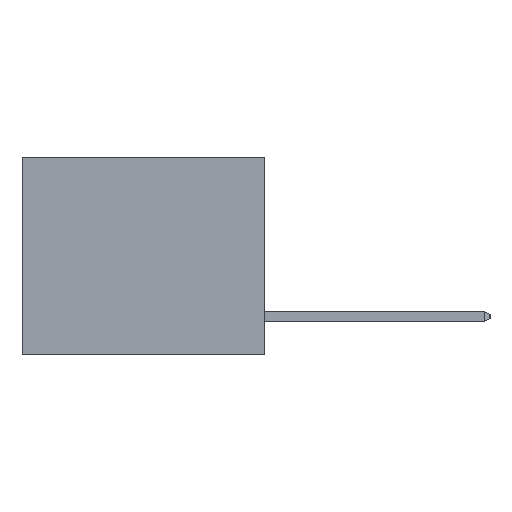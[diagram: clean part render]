
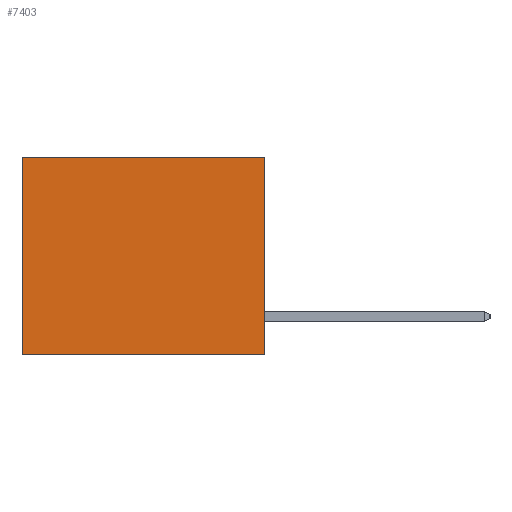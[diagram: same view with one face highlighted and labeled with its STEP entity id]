
A CAD part, left-side view. The second image highlights one B-rep face of the part: STEP entity #7403.
In plain terms, the highlighted planar face has unit normal (-1, 0, 0).
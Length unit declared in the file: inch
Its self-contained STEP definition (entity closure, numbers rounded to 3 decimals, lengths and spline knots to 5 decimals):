
#246 = AXIS2_PLACEMENT_3D ( 'NONE', #17923, #2423, #8556 ) ;
#753 = VECTOR ( 'NONE', #1639, 39.37008 ) ;
#1365 = CARTESIAN_POINT ( 'NONE',  ( 0.3165, 0., -0.49 ) ) ;
#1639 = DIRECTION ( 'NONE',  ( 0., 1., 0. ) ) ;
#1833 = CARTESIAN_POINT ( 'NONE',  ( 0.3165, 0., 0. ) ) ;
#2423 = DIRECTION ( 'NONE',  ( 1., 0., 0. ) ) ;
#2845 = CARTESIAN_POINT ( 'NONE',  ( 0.3165, 0., 0. ) ) ;
#3316 = CARTESIAN_POINT ( 'NONE',  ( 0.3165, 0.6, -0.49 ) ) ;
#3956 = VECTOR ( 'NONE', #10440, 39.37008 ) ;
#4704 = CARTESIAN_POINT ( 'NONE',  ( 0.3165, 0., -0.49 ) ) ;
#4845 = VERTEX_POINT ( 'NONE', #12068 ) ;
#5473 = PLANE ( 'NONE',  #246 ) ;
#5588 = ORIENTED_EDGE ( 'NONE', *, *, #15185, .T. ) ;
#6753 = EDGE_CURVE ( 'NONE', #7168, #4845, #12790, .T. ) ;
#7168 = VERTEX_POINT ( 'NONE', #2845 ) ;
#7403 = ADVANCED_FACE ( 'NONE', ( #8034 ), #5473, .F. ) ;
#7908 = LINE ( 'NONE', #1365, #19827 ) ;
#8034 = FACE_OUTER_BOUND ( 'NONE', #8090, .T. ) ;
#8090 = EDGE_LOOP ( 'NONE', ( #8591, #9976, #17441, #5588 ) ) ;
#8556 = DIRECTION ( 'NONE',  ( 0., 0., -1. ) ) ;
#8591 = ORIENTED_EDGE ( 'NONE', *, *, #18646, .T. ) ;
#8878 = CARTESIAN_POINT ( 'NONE',  ( 0.3165, 0.6, -0.49 ) ) ;
#9976 = ORIENTED_EDGE ( 'NONE', *, *, #17591, .F. ) ;
#10440 = DIRECTION ( 'NONE',  ( 0., 0., -1. ) ) ;
#12068 = CARTESIAN_POINT ( 'NONE',  ( 0.3165, 0., -0.49 ) ) ;
#12761 = VERTEX_POINT ( 'NONE', #3316 ) ;
#12790 = LINE ( 'NONE', #4704, #16690 ) ;
#15185 = EDGE_CURVE ( 'NONE', #7168, #17456, #17766, .T. ) ;
#15728 = DIRECTION ( 'NONE',  ( 0., 0., -1. ) ) ;
#15958 = CARTESIAN_POINT ( 'NONE',  ( 0.3165, 0.6, 0. ) ) ;
#16690 = VECTOR ( 'NONE', #15728, 39.37008 ) ;
#17441 = ORIENTED_EDGE ( 'NONE', *, *, #6753, .F. ) ;
#17456 = VERTEX_POINT ( 'NONE', #15958 ) ;
#17591 = EDGE_CURVE ( 'NONE', #4845, #12761, #7908, .T. ) ;
#17766 = LINE ( 'NONE', #1833, #753 ) ;
#17923 = CARTESIAN_POINT ( 'NONE',  ( 0.3165, 0., -0.49 ) ) ;
#18646 = EDGE_CURVE ( 'NONE', #17456, #12761, #18791, .T. ) ;
#18791 = LINE ( 'NONE', #8878, #3956 ) ;
#19827 = VECTOR ( 'NONE', #19908, 39.37008 ) ;
#19908 = DIRECTION ( 'NONE',  ( 0., 1., 0. ) ) ;
